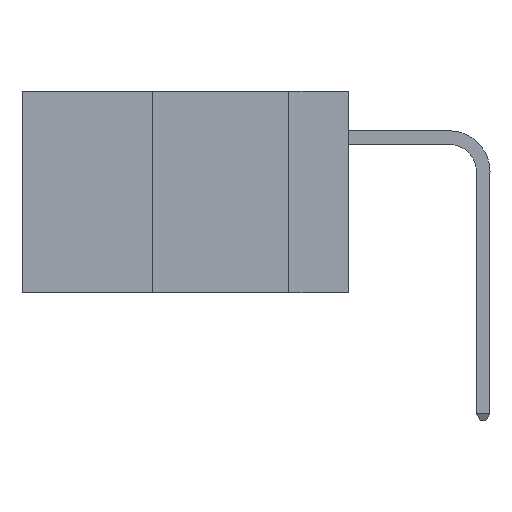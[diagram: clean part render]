
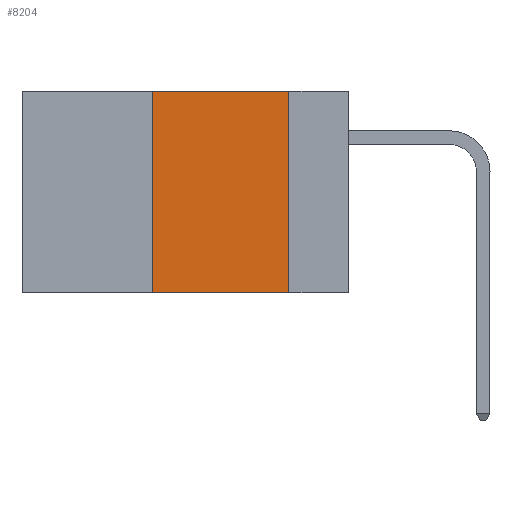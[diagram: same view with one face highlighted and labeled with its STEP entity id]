
A CAD part, left-side view. The second image highlights one B-rep face of the part: STEP entity #8204.
In plain terms, the highlighted planar face has unit normal (-1, 0, 0).
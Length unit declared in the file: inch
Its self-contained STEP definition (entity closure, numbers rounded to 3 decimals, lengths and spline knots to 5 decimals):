
#384 = DIRECTION ( 'NONE',  ( 0., 0., -1. ) ) ;
#464 = LINE ( 'NONE', #2319, #6156 ) ;
#1403 = EDGE_CURVE ( 'NONE', #10317, #1770, #1407, .T. ) ;
#1407 = LINE ( 'NONE', #10661, #13051 ) ;
#1465 = EDGE_CURVE ( 'NONE', #4739, #12197, #12719, .T. ) ;
#1770 = VERTEX_POINT ( 'NONE', #13867 ) ;
#1877 = VECTOR ( 'NONE', #7717, 39.37008 ) ;
#2199 = CARTESIAN_POINT ( 'NONE',  ( 0., 0.11, 0. ) ) ;
#2278 = DIRECTION ( 'NONE',  ( 0., 0., 1. ) ) ;
#2319 = CARTESIAN_POINT ( 'NONE',  ( 0., 0.36, 0. ) ) ;
#2665 = CARTESIAN_POINT ( 'NONE',  ( 0., 0.36, -0.37 ) ) ;
#3532 = CARTESIAN_POINT ( 'NONE',  ( 0., 0.6, 0. ) ) ;
#3673 = ORIENTED_EDGE ( 'NONE', *, *, #10003, .F. ) ;
#3705 = EDGE_CURVE ( 'NONE', #4739, #10317, #464, .T. ) ;
#3954 = CARTESIAN_POINT ( 'NONE',  ( 0., 0.11, -0.37 ) ) ;
#4739 = VERTEX_POINT ( 'NONE', #2665 ) ;
#5467 = LINE ( 'NONE', #2199, #8652 ) ;
#5550 = AXIS2_PLACEMENT_3D ( 'NONE', #3532, #11042, #384 ) ;
#6156 = VECTOR ( 'NONE', #2278, 39.37008 ) ;
#6389 = ORIENTED_EDGE ( 'NONE', *, *, #1403, .F. ) ;
#6702 = PLANE ( 'NONE',  #5550 ) ;
#7014 = CARTESIAN_POINT ( 'NONE',  ( 0., 0.6, -0.37 ) ) ;
#7655 = FACE_OUTER_BOUND ( 'NONE', #10263, .T. ) ;
#7717 = DIRECTION ( 'NONE',  ( 0., -1., 0. ) ) ;
#8091 = DIRECTION ( 'NONE',  ( 0., -1., 0. ) ) ;
#8204 = ADVANCED_FACE ( 'NONE', ( #7655 ), #6702, .F. ) ;
#8652 = VECTOR ( 'NONE', #11810, 39.37008 ) ;
#10003 = EDGE_CURVE ( 'NONE', #1770, #12197, #5467, .T. ) ;
#10263 = EDGE_LOOP ( 'NONE', ( #3673, #6389, #13235, #13770 ) ) ;
#10317 = VERTEX_POINT ( 'NONE', #13574 ) ;
#10661 = CARTESIAN_POINT ( 'NONE',  ( 0., 0.6, 0. ) ) ;
#11042 = DIRECTION ( 'NONE',  ( 1., 0., 0. ) ) ;
#11810 = DIRECTION ( 'NONE',  ( 0., 0., -1. ) ) ;
#12197 = VERTEX_POINT ( 'NONE', #3954 ) ;
#12719 = LINE ( 'NONE', #7014, #1877 ) ;
#13051 = VECTOR ( 'NONE', #8091, 39.37008 ) ;
#13235 = ORIENTED_EDGE ( 'NONE', *, *, #3705, .F. ) ;
#13574 = CARTESIAN_POINT ( 'NONE',  ( 0., 0.36, 0. ) ) ;
#13770 = ORIENTED_EDGE ( 'NONE', *, *, #1465, .T. ) ;
#13867 = CARTESIAN_POINT ( 'NONE',  ( 0., 0.11, 0. ) ) ;
